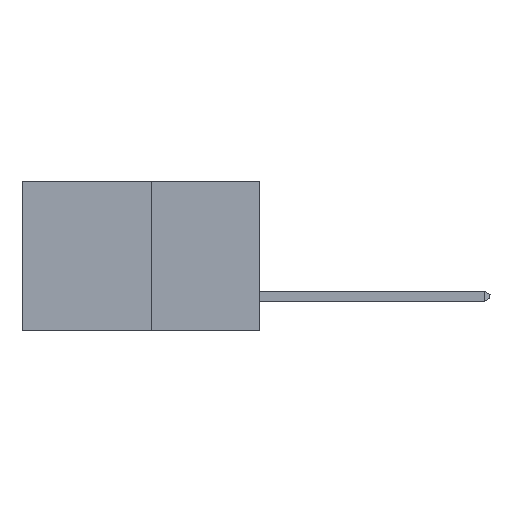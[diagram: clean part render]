
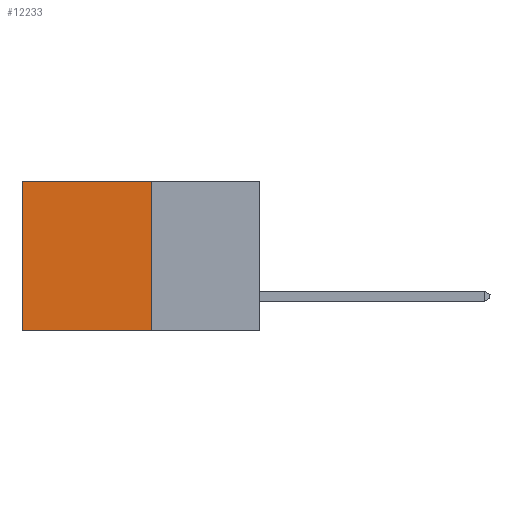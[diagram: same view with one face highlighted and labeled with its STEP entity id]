
A CAD part, left-side view. The second image highlights one B-rep face of the part: STEP entity #12233.
In plain terms, the highlighted planar face has unit normal (-1, 0, 0).
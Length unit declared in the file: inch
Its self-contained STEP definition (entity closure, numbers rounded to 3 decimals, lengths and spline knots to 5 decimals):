
#165 = CARTESIAN_POINT ( 'NONE',  ( 0.277, 0.27, -0.37 ) ) ;
#608 = ORIENTED_EDGE ( 'NONE', *, *, #634, .T. ) ;
#634 = EDGE_CURVE ( 'NONE', #5002, #15486, #18803, .T. ) ;
#1705 = CARTESIAN_POINT ( 'NONE',  ( 0.277, 0.27, 0. ) ) ;
#1818 = DIRECTION ( 'NONE',  ( 0., 1., 0. ) ) ;
#2610 = LINE ( 'NONE', #165, #11268 ) ;
#4225 = ORIENTED_EDGE ( 'NONE', *, *, #4858, .T. ) ;
#4858 = EDGE_CURVE ( 'NONE', #12471, #5002, #19498, .T. ) ;
#5002 = VERTEX_POINT ( 'NONE', #5375 ) ;
#5375 = CARTESIAN_POINT ( 'NONE',  ( 0.277, 0.59, 0. ) ) ;
#7946 = DIRECTION ( 'NONE',  ( 0., 0., -1. ) ) ;
#8310 = DIRECTION ( 'NONE',  ( 0., 1., 0. ) ) ;
#8441 = ORIENTED_EDGE ( 'NONE', *, *, #17765, .F. ) ;
#8688 = LINE ( 'NONE', #15963, #18165 ) ;
#9080 = CARTESIAN_POINT ( 'NONE',  ( 0.277, 0.27, -0.37 ) ) ;
#9162 = ORIENTED_EDGE ( 'NONE', *, *, #10442, .F. ) ;
#9287 = PLANE ( 'NONE',  #10634 ) ;
#9346 = CARTESIAN_POINT ( 'NONE',  ( 0.277, 0.59, -0.37 ) ) ;
#9357 = DIRECTION ( 'NONE',  ( 1., 0., 0. ) ) ;
#9944 = VECTOR ( 'NONE', #8310, 39.37008 ) ;
#10442 = EDGE_CURVE ( 'NONE', #11495, #15486, #2610, .T. ) ;
#10634 = AXIS2_PLACEMENT_3D ( 'NONE', #10902, #9357, #20595 ) ;
#10902 = CARTESIAN_POINT ( 'NONE',  ( 0.277, 0.27, -0.37 ) ) ;
#11268 = VECTOR ( 'NONE', #1818, 39.37008 ) ;
#11455 = CARTESIAN_POINT ( 'NONE',  ( 0.277, 0.27, 0. ) ) ;
#11495 = VERTEX_POINT ( 'NONE', #9080 ) ;
#11514 = DIRECTION ( 'NONE',  ( 0., 0., -1. ) ) ;
#12233 = ADVANCED_FACE ( 'NONE', ( #18723 ), #9287, .F. ) ;
#12471 = VERTEX_POINT ( 'NONE', #11455 ) ;
#15486 = VERTEX_POINT ( 'NONE', #16793 ) ;
#15717 = EDGE_LOOP ( 'NONE', ( #608, #9162, #8441, #4225 ) ) ;
#15963 = CARTESIAN_POINT ( 'NONE',  ( 0.277, 0.27, -0.37 ) ) ;
#16793 = CARTESIAN_POINT ( 'NONE',  ( 0.277, 0.59, -0.37 ) ) ;
#17765 = EDGE_CURVE ( 'NONE', #12471, #11495, #8688, .T. ) ;
#18165 = VECTOR ( 'NONE', #7946, 39.37008 ) ;
#18292 = VECTOR ( 'NONE', #11514, 39.37008 ) ;
#18723 = FACE_OUTER_BOUND ( 'NONE', #15717, .T. ) ;
#18803 = LINE ( 'NONE', #9346, #18292 ) ;
#19498 = LINE ( 'NONE', #1705, #9944 ) ;
#20595 = DIRECTION ( 'NONE',  ( 0., 0., -1. ) ) ;
